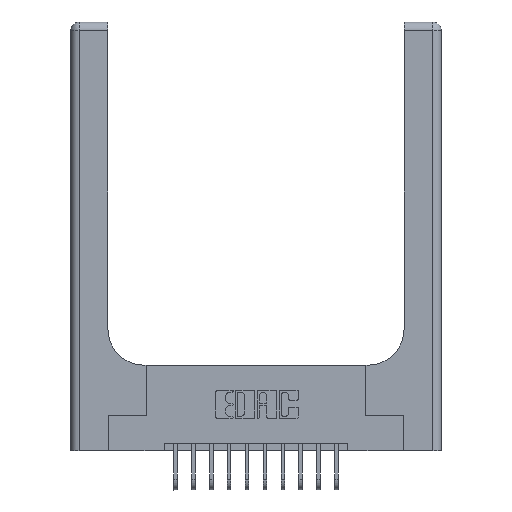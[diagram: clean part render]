
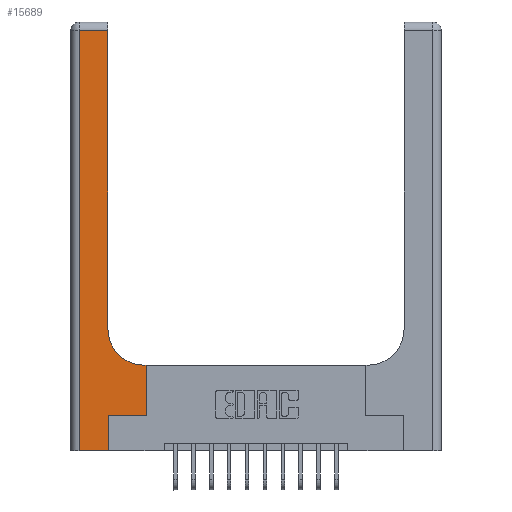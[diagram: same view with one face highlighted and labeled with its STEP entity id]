
A CAD part, top view. The second image highlights one B-rep face of the part: STEP entity #15689.
In plain terms, the highlighted planar face has unit normal (0, 0, 1).
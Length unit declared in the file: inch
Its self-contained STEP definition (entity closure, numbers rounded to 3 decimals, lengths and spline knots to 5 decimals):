
#213 = DIRECTION ( 'NONE',  ( 1., 0., 0. ) ) ;
#273 = CARTESIAN_POINT ( 'NONE',  ( 0.528, 0.25, 0.37 ) ) ;
#515 = PLANE ( 'NONE',  #8730 ) ;
#635 = LINE ( 'NONE', #8028, #2907 ) ;
#797 = DIRECTION ( 'NONE',  ( -1., 0., 0. ) ) ;
#1281 = EDGE_LOOP ( 'NONE', ( #1469, #6841, #8021, #2064, #7581, #14625, #15575, #2092, #4171 ) ) ;
#1393 = CARTESIAN_POINT ( 'NONE',  ( 0.51, 0.6, 0.37 ) ) ;
#1441 = CARTESIAN_POINT ( 'NONE',  ( 0.26, 0.85, 0.37 ) ) ;
#1469 = ORIENTED_EDGE ( 'NONE', *, *, #15407, .T. ) ;
#1477 = LINE ( 'NONE', #9274, #8944 ) ;
#1804 = DIRECTION ( 'NONE',  ( 0., 1., 0. ) ) ;
#2064 = ORIENTED_EDGE ( 'NONE', *, *, #7675, .T. ) ;
#2092 = ORIENTED_EDGE ( 'NONE', *, *, #14199, .T. ) ;
#2345 = VECTOR ( 'NONE', #4071, 39.37008 ) ;
#2493 = DIRECTION ( 'NONE',  ( 0., 1., 0. ) ) ;
#2564 = LINE ( 'NONE', #2727, #3102 ) ;
#2727 = CARTESIAN_POINT ( 'NONE',  ( 0.06, 3., 0.37 ) ) ;
#2907 = VECTOR ( 'NONE', #797, 39.37008 ) ;
#3038 = DIRECTION ( 'NONE',  ( -1., 0., 0. ) ) ;
#3102 = VECTOR ( 'NONE', #8961, 39.37008 ) ;
#3658 = VECTOR ( 'NONE', #1804, 39.37008 ) ;
#3702 = CARTESIAN_POINT ( 'NONE',  ( 0.265, 0., 0.37 ) ) ;
#3997 = LINE ( 'NONE', #5141, #2345 ) ;
#4071 = DIRECTION ( 'NONE',  ( 1., 0., 0. ) ) ;
#4171 = ORIENTED_EDGE ( 'NONE', *, *, #5367, .T. ) ;
#4271 = CARTESIAN_POINT ( 'NONE',  ( 0., 3., 0.37 ) ) ;
#4435 = CARTESIAN_POINT ( 'NONE',  ( 0.265, 0., 0.37 ) ) ;
#4798 = CARTESIAN_POINT ( 'NONE',  ( 0.528, 0.25, 0.37 ) ) ;
#5141 = CARTESIAN_POINT ( 'NONE',  ( 0., 0., 0.37 ) ) ;
#5360 = VERTEX_POINT ( 'NONE', #1441 ) ;
#5367 = EDGE_CURVE ( 'NONE', #7654, #5360, #15155, .T. ) ;
#5502 = FACE_OUTER_BOUND ( 'NONE', #1281, .T. ) ;
#5730 = VECTOR ( 'NONE', #7580, 39.37008 ) ;
#5732 = CARTESIAN_POINT ( 'NONE',  ( 0.06, 2.94, 0.37 ) ) ;
#5752 = VERTEX_POINT ( 'NONE', #4435 ) ;
#6433 = CARTESIAN_POINT ( 'NONE',  ( 0.51, 0.85, 0.37 ) ) ;
#6745 = VERTEX_POINT ( 'NONE', #9819 ) ;
#6841 = ORIENTED_EDGE ( 'NONE', *, *, #13549, .T. ) ;
#7425 = VERTEX_POINT ( 'NONE', #5732 ) ;
#7509 = CARTESIAN_POINT ( 'NONE',  ( 0.26, 3., 0.37 ) ) ;
#7580 = DIRECTION ( 'NONE',  ( 0., 1., 0. ) ) ;
#7581 = ORIENTED_EDGE ( 'NONE', *, *, #11598, .T. ) ;
#7654 = VERTEX_POINT ( 'NONE', #1393 ) ;
#7675 = EDGE_CURVE ( 'NONE', #13946, #5752, #3997, .T. ) ;
#7762 = LINE ( 'NONE', #12860, #15960 ) ;
#8021 = ORIENTED_EDGE ( 'NONE', *, *, #11634, .T. ) ;
#8028 = CARTESIAN_POINT ( 'NONE',  ( 0., 2.94, 0.37 ) ) ;
#8730 = AXIS2_PLACEMENT_3D ( 'NONE', #4271, #14318, #3038 ) ;
#8731 = LINE ( 'NONE', #3702, #5730 ) ;
#8874 = CARTESIAN_POINT ( 'NONE',  ( 0.26, 2.94, 0.37 ) ) ;
#8944 = VECTOR ( 'NONE', #9101, 39.37008 ) ;
#8961 = DIRECTION ( 'NONE',  ( 0., -1., 0. ) ) ;
#9032 = VERTEX_POINT ( 'NONE', #8874 ) ;
#9101 = DIRECTION ( 'NONE',  ( -1., 0., 0. ) ) ;
#9274 = CARTESIAN_POINT ( 'NONE',  ( 0.26, 0.6, 0.37 ) ) ;
#9819 = CARTESIAN_POINT ( 'NONE',  ( 0.528, 0.6, 0.37 ) ) ;
#10056 = VECTOR ( 'NONE', #2493, 39.37008 ) ;
#10180 = AXIS2_PLACEMENT_3D ( 'NONE', #6433, #11469, #213 ) ;
#11199 = VERTEX_POINT ( 'NONE', #4798 ) ;
#11278 = EDGE_CURVE ( 'NONE', #14327, #11199, #7762, .T. ) ;
#11469 = DIRECTION ( 'NONE',  ( 0., 0., -1. ) ) ;
#11598 = EDGE_CURVE ( 'NONE', #5752, #14327, #8731, .T. ) ;
#11634 = EDGE_CURVE ( 'NONE', #7425, #13946, #2564, .T. ) ;
#11852 = LINE ( 'NONE', #273, #3658 ) ;
#12209 = LINE ( 'NONE', #7509, #10056 ) ;
#12247 = CARTESIAN_POINT ( 'NONE',  ( 0.265, 0.25, 0.37 ) ) ;
#12542 = EDGE_CURVE ( 'NONE', #11199, #6745, #11852, .T. ) ;
#12860 = CARTESIAN_POINT ( 'NONE',  ( 0.265, 0.25, 0.37 ) ) ;
#13413 = CARTESIAN_POINT ( 'NONE',  ( 0.06, 0., 0.37 ) ) ;
#13549 = EDGE_CURVE ( 'NONE', #9032, #7425, #635, .T. ) ;
#13946 = VERTEX_POINT ( 'NONE', #13413 ) ;
#14098 = DIRECTION ( 'NONE',  ( 1., 0., 0. ) ) ;
#14199 = EDGE_CURVE ( 'NONE', #6745, #7654, #1477, .T. ) ;
#14318 = DIRECTION ( 'NONE',  ( 0., 0., -1. ) ) ;
#14327 = VERTEX_POINT ( 'NONE', #12247 ) ;
#14625 = ORIENTED_EDGE ( 'NONE', *, *, #11278, .T. ) ;
#15155 = CIRCLE ( 'NONE', #10180, 0.25 ) ;
#15407 = EDGE_CURVE ( 'NONE', #5360, #9032, #12209, .T. ) ;
#15575 = ORIENTED_EDGE ( 'NONE', *, *, #12542, .T. ) ;
#15689 = ADVANCED_FACE ( 'NONE', ( #5502 ), #515, .F. ) ;
#15960 = VECTOR ( 'NONE', #14098, 39.37008 ) ;
